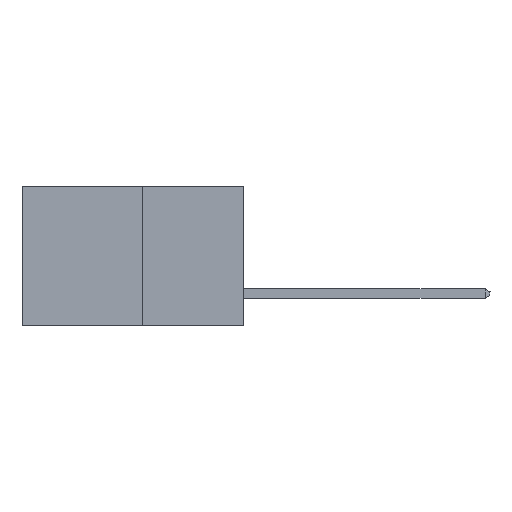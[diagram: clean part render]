
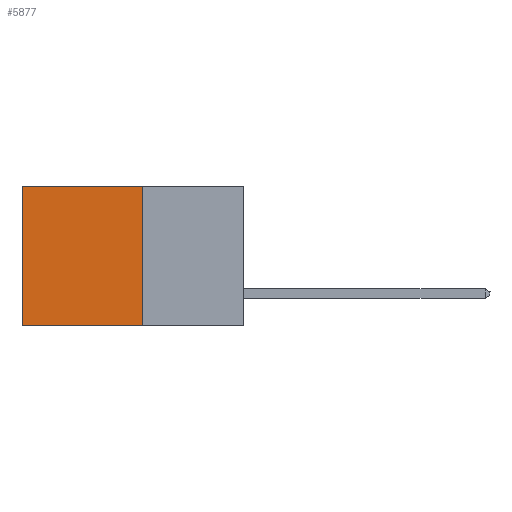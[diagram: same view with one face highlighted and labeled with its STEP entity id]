
A CAD part, left-side view. The second image highlights one B-rep face of the part: STEP entity #5877.
In plain terms, the highlighted planar face has unit normal (-1, 0, 0).
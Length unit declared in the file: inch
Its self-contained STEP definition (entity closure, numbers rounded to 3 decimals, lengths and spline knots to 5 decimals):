
#417 = CARTESIAN_POINT ( 'NONE',  ( 0.277, 0.59, -0.37 ) ) ;
#429 = ORIENTED_EDGE ( 'NONE', *, *, #6025, .F. ) ;
#743 = AXIS2_PLACEMENT_3D ( 'NONE', #9373, #9313, #9310 ) ;
#1124 = CARTESIAN_POINT ( 'NONE',  ( 0.277, 0.27, 0. ) ) ;
#1213 = EDGE_CURVE ( 'NONE', #7496, #2773, #8101, .T. ) ;
#1285 = EDGE_CURVE ( 'NONE', #7496, #1339, #5071, .T. ) ;
#1339 = VERTEX_POINT ( 'NONE', #2852 ) ;
#2773 = VERTEX_POINT ( 'NONE', #11356 ) ;
#2802 = ORIENTED_EDGE ( 'NONE', *, *, #1213, .F. ) ;
#2813 = VECTOR ( 'NONE', #6844, 39.37008 ) ;
#2852 = CARTESIAN_POINT ( 'NONE',  ( 0.277, 0.59, 0. ) ) ;
#3131 = VECTOR ( 'NONE', #9853, 39.37008 ) ;
#3399 = VECTOR ( 'NONE', #7155, 39.37008 ) ;
#3526 = CARTESIAN_POINT ( 'NONE',  ( 0.277, 0.59, -0.37 ) ) ;
#4562 = ORIENTED_EDGE ( 'NONE', *, *, #7955, .T. ) ;
#4828 = DIRECTION ( 'NONE',  ( 0., 1., 0. ) ) ;
#5071 = LINE ( 'NONE', #8700, #11956 ) ;
#5623 = ORIENTED_EDGE ( 'NONE', *, *, #1285, .T. ) ;
#5877 = ADVANCED_FACE ( 'NONE', ( #9195 ), #9516, .F. ) ;
#6025 = EDGE_CURVE ( 'NONE', #2773, #11019, #10205, .T. ) ;
#6782 = EDGE_LOOP ( 'NONE', ( #4562, #429, #2802, #5623 ) ) ;
#6844 = DIRECTION ( 'NONE',  ( 0., 1., 0. ) ) ;
#7015 = CARTESIAN_POINT ( 'NONE',  ( 0.277, 0.27, -0.37 ) ) ;
#7155 = DIRECTION ( 'NONE',  ( 0., 0., -1. ) ) ;
#7496 = VERTEX_POINT ( 'NONE', #1124 ) ;
#7955 = EDGE_CURVE ( 'NONE', #1339, #11019, #8060, .T. ) ;
#8060 = LINE ( 'NONE', #417, #3399 ) ;
#8101 = LINE ( 'NONE', #9552, #3131 ) ;
#8700 = CARTESIAN_POINT ( 'NONE',  ( 0.277, 0.27, 0. ) ) ;
#9195 = FACE_OUTER_BOUND ( 'NONE', #6782, .T. ) ;
#9310 = DIRECTION ( 'NONE',  ( 0., 0., -1. ) ) ;
#9313 = DIRECTION ( 'NONE',  ( 1., 0., 0. ) ) ;
#9373 = CARTESIAN_POINT ( 'NONE',  ( 0.277, 0.27, -0.37 ) ) ;
#9516 = PLANE ( 'NONE',  #743 ) ;
#9552 = CARTESIAN_POINT ( 'NONE',  ( 0.277, 0.27, -0.37 ) ) ;
#9853 = DIRECTION ( 'NONE',  ( 0., 0., -1. ) ) ;
#10205 = LINE ( 'NONE', #7015, #2813 ) ;
#11019 = VERTEX_POINT ( 'NONE', #3526 ) ;
#11356 = CARTESIAN_POINT ( 'NONE',  ( 0.277, 0.27, -0.37 ) ) ;
#11956 = VECTOR ( 'NONE', #4828, 39.37008 ) ;
